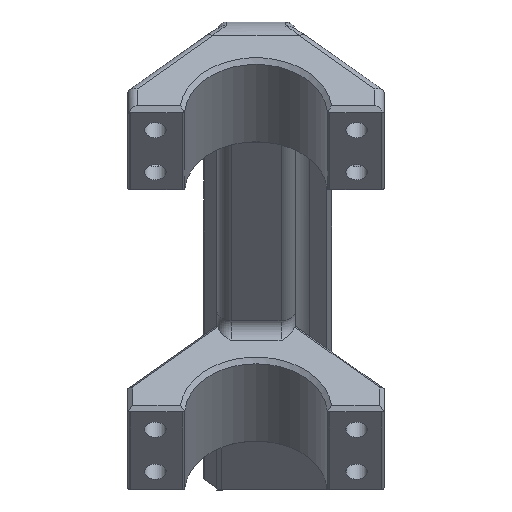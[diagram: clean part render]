
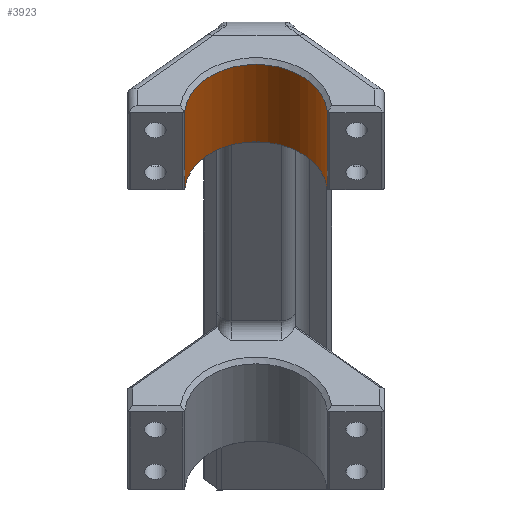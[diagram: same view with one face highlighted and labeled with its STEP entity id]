
A CAD part, top view. The second image highlights one B-rep face of the part: STEP entity #3923.
In plain terms, the highlighted cylindrical face has radius 15 mm (diameter 30 mm), a partial arc.
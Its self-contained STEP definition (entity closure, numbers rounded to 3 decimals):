
#55=CYLINDRICAL_SURFACE('',#4209,15.);
#88=CIRCLE('',#4090,15.);
#106=CIRCLE('',#4208,15.);
#296=FACE_OUTER_BOUND('',#517,.T.);
#517=EDGE_LOOP('',(#3139,#3140,#3141,#3142));
#761=LINE('',#5701,#1203);
#767=LINE('',#5732,#1209);
#1203=VECTOR('',#4518,10.);
#1209=VECTOR('',#4544,10.);
#1661=VERTEX_POINT('',#5664);
#1662=VERTEX_POINT('',#5673);
#1666=VERTEX_POINT('',#5692);
#1675=VERTEX_POINT('',#5731);
#2054=EDGE_CURVE('',#1662,#1661,#88,.T.);
#2060=EDGE_CURVE('',#1661,#1666,#761,.T.);
#2073=EDGE_CURVE('',#1675,#1662,#767,.T.);
#2307=EDGE_CURVE('',#1666,#1675,#106,.T.);
#3139=ORIENTED_EDGE('',*,*,#2060,.T.);
#3140=ORIENTED_EDGE('',*,*,#2307,.T.);
#3141=ORIENTED_EDGE('',*,*,#2073,.T.);
#3142=ORIENTED_EDGE('',*,*,#2054,.T.);
#3923=ADVANCED_FACE('',(#296),#55,.F.);
#4090=AXIS2_PLACEMENT_3D('',#5674,#4511,#4512);
#4208=AXIS2_PLACEMENT_3D('',#6354,#4942,#4943);
#4209=AXIS2_PLACEMENT_3D('',#6355,#4944,#4945);
#4511=DIRECTION('center_axis',(0.,0.707,
0.707));
#4512=DIRECTION('ref_axis',(-1.,0.,0.));
#4518=DIRECTION('',(0.,-0.707,-0.707));
#4544=DIRECTION('',(0.,0.707,0.707));
#4942=DIRECTION('center_axis',(0.,-0.707,
-0.707));
#4943=DIRECTION('ref_axis',(-1.,0.,0.));
#4944=DIRECTION('center_axis',(0.,-0.707,
-0.707));
#4945=DIRECTION('ref_axis',(-1.,0.,0.));
#5664=CARTESIAN_POINT('',(-14.952,94.158,130.368));
#5673=CARTESIAN_POINT('',(14.952,94.158,130.368));
#5674=CARTESIAN_POINT('Origin',(0.,93.308,
131.218));
#5692=CARTESIAN_POINT('',(-14.952,77.894,114.105));
#5701=CARTESIAN_POINT('',(-14.952,14.255,50.465));
#5731=CARTESIAN_POINT('',(14.952,77.894,114.105));
#5732=CARTESIAN_POINT('',(14.952,14.255,50.465));
#6354=CARTESIAN_POINT('Origin',(0.,77.044,
114.955));
#6355=CARTESIAN_POINT('Origin',(0.,13.405,51.315));
